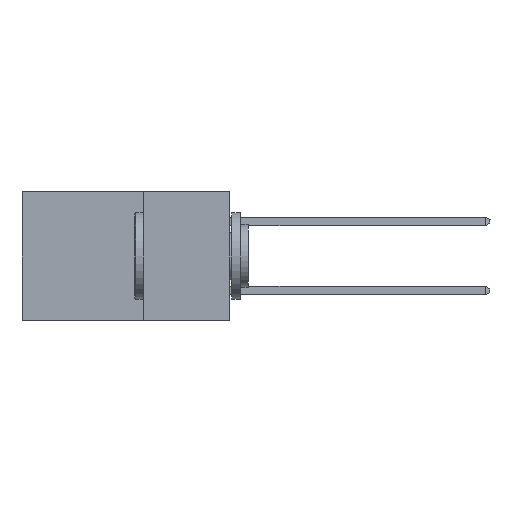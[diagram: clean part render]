
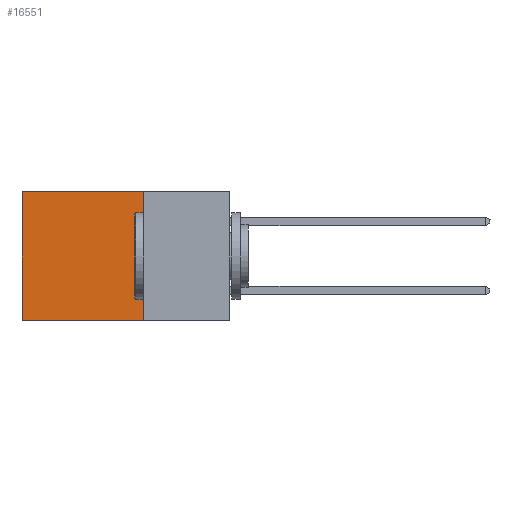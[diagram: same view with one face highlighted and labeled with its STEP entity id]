
A CAD part, left-side view. The second image highlights one B-rep face of the part: STEP entity #16551.
In plain terms, the highlighted planar face has unit normal (-1, 0, 0).
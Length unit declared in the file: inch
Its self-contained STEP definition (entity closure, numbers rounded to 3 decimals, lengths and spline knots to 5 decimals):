
#47 = ORIENTED_EDGE ( 'NONE', *, *, #19472, .T. ) ;
#67 = CARTESIAN_POINT ( 'NONE',  ( 0.2615, 0.25, -0.37 ) ) ;
#624 = VECTOR ( 'NONE', #16228, 39.37008 ) ;
#712 = CARTESIAN_POINT ( 'NONE',  ( 0.2615, 0.25, -0.37 ) ) ;
#1504 = CARTESIAN_POINT ( 'NONE',  ( 0.2615, 0.25, 0. ) ) ;
#1659 = VECTOR ( 'NONE', #9875, 39.37008 ) ;
#1676 = VECTOR ( 'NONE', #11144, 39.37008 ) ;
#2014 = VERTEX_POINT ( 'NONE', #19576 ) ;
#2433 = EDGE_CURVE ( 'NONE', #20463, #2014, #19434, .T. ) ;
#2781 = VECTOR ( 'NONE', #20929, 39.37008 ) ;
#2889 = CARTESIAN_POINT ( 'NONE',  ( 0.2615, 0.25, 0. ) ) ;
#4959 = ORIENTED_EDGE ( 'NONE', *, *, #19038, .F. ) ;
#6295 = FACE_OUTER_BOUND ( 'NONE', #9682, .T. ) ;
#6482 = LINE ( 'NONE', #17381, #2781 ) ;
#8776 = VERTEX_POINT ( 'NONE', #1504 ) ;
#8980 = AXIS2_PLACEMENT_3D ( 'NONE', #712, #18739, #22404 ) ;
#9116 = CARTESIAN_POINT ( 'NONE',  ( 0.2615, 0.6, -0.37 ) ) ;
#9351 = LINE ( 'NONE', #9116, #1676 ) ;
#9492 = PLANE ( 'NONE',  #8980 ) ;
#9682 = EDGE_LOOP ( 'NONE', ( #17462, #11477, #4959, #47 ) ) ;
#9875 = DIRECTION ( 'NONE',  ( 0., 1., 0. ) ) ;
#11144 = DIRECTION ( 'NONE',  ( 0., 0., -1. ) ) ;
#11477 = ORIENTED_EDGE ( 'NONE', *, *, #2433, .F. ) ;
#15565 = CARTESIAN_POINT ( 'NONE',  ( 0.2615, 0.6, 0. ) ) ;
#16228 = DIRECTION ( 'NONE',  ( 0., 1., 0. ) ) ;
#16551 = ADVANCED_FACE ( 'NONE', ( #6295 ), #9492, .F. ) ;
#17381 = CARTESIAN_POINT ( 'NONE',  ( 0.2615, 0.25, -0.37 ) ) ;
#17462 = ORIENTED_EDGE ( 'NONE', *, *, #21764, .T. ) ;
#18115 = VERTEX_POINT ( 'NONE', #15565 ) ;
#18739 = DIRECTION ( 'NONE',  ( 1., 0., 0. ) ) ;
#19038 = EDGE_CURVE ( 'NONE', #8776, #20463, #6482, .T. ) ;
#19434 = LINE ( 'NONE', #19778, #624 ) ;
#19472 = EDGE_CURVE ( 'NONE', #8776, #18115, #22918, .T. ) ;
#19576 = CARTESIAN_POINT ( 'NONE',  ( 0.2615, 0.6, -0.37 ) ) ;
#19778 = CARTESIAN_POINT ( 'NONE',  ( 0.2615, 0.25, -0.37 ) ) ;
#20463 = VERTEX_POINT ( 'NONE', #67 ) ;
#20929 = DIRECTION ( 'NONE',  ( 0., 0., -1. ) ) ;
#21764 = EDGE_CURVE ( 'NONE', #18115, #2014, #9351, .T. ) ;
#22404 = DIRECTION ( 'NONE',  ( 0., 0., -1. ) ) ;
#22918 = LINE ( 'NONE', #2889, #1659 ) ;
